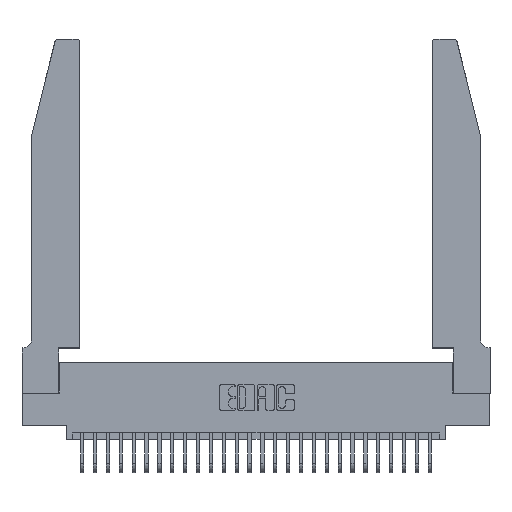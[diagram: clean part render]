
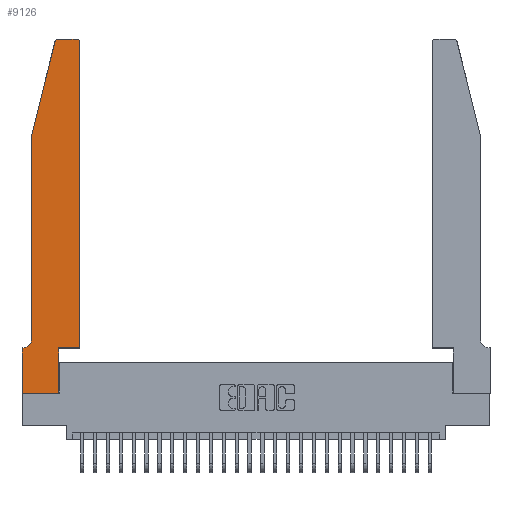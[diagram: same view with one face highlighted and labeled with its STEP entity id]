
A CAD part, top view. The second image highlights one B-rep face of the part: STEP entity #9126.
In plain terms, the highlighted planar face has unit normal (0, 0, 1).
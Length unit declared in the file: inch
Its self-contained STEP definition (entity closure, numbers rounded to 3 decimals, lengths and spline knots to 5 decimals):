
#20 = VECTOR ( 'NONE', #21429, 39.37008 ) ;
#166 = CARTESIAN_POINT ( 'NONE',  ( 0.284, 2.72, 0.37 ) ) ;
#540 = AXIS2_PLACEMENT_3D ( 'NONE', #166, #8974, #23031 ) ;
#569 = DIRECTION ( 'NONE',  ( -1., 0., 0. ) ) ;
#892 = LINE ( 'NONE', #29978, #26623 ) ;
#1623 = CIRCLE ( 'NONE', #21511, 0.03 ) ;
#2036 = CIRCLE ( 'NONE', #540, 0.03 ) ;
#2451 = DIRECTION ( 'NONE',  ( 0., 1., 0. ) ) ;
#2633 = EDGE_LOOP ( 'NONE', ( #7762, #2646, #11459, #7967, #24543, #28884, #22495, #23406, #10950, #25258, #8708, #3749 ) ) ;
#2646 = ORIENTED_EDGE ( 'NONE', *, *, #6330, .T. ) ;
#2944 = EDGE_CURVE ( 'NONE', #3368, #30185, #22848, .T. ) ;
#3368 = VERTEX_POINT ( 'NONE', #3520 ) ;
#3520 = CARTESIAN_POINT ( 'NONE',  ( 0.0755, 0.42, 0.37 ) ) ;
#3694 = LINE ( 'NONE', #16922, #20 ) ;
#3749 = ORIENTED_EDGE ( 'NONE', *, *, #21285, .T. ) ;
#3781 = CARTESIAN_POINT ( 'NONE',  ( 0.4505, 2.72, 0.37 ) ) ;
#3978 = VECTOR ( 'NONE', #569, 39.37008 ) ;
#5810 = EDGE_CURVE ( 'NONE', #25980, #11732, #6088, .T. ) ;
#6088 = LINE ( 'NONE', #26277, #10878 ) ;
#6330 = EDGE_CURVE ( 'NONE', #10317, #6847, #2036, .T. ) ;
#6740 = VECTOR ( 'NONE', #25103, 39.37008 ) ;
#6847 = VERTEX_POINT ( 'NONE', #18614 ) ;
#6936 = EDGE_CURVE ( 'NONE', #20469, #14770, #15983, .T. ) ;
#7747 = CARTESIAN_POINT ( 'NONE',  ( 0.2605, 2.75, 0.37 ) ) ;
#7762 = ORIENTED_EDGE ( 'NONE', *, *, #21442, .T. ) ;
#7824 = LINE ( 'NONE', #16456, #25850 ) ;
#7967 = ORIENTED_EDGE ( 'NONE', *, *, #21845, .T. ) ;
#8351 = VERTEX_POINT ( 'NONE', #26873 ) ;
#8708 = ORIENTED_EDGE ( 'NONE', *, *, #12063, .T. ) ;
#8974 = DIRECTION ( 'NONE',  ( 0., 0., 1. ) ) ;
#9126 = ADVANCED_FACE ( 'NONE', ( #10341 ), #14362, .T. ) ;
#9765 = CARTESIAN_POINT ( 'NONE',  ( 0.0055, 0.35, 0.37 ) ) ;
#10127 = EDGE_CURVE ( 'NONE', #14770, #8351, #7824, .T. ) ;
#10317 = VERTEX_POINT ( 'NONE', #12602 ) ;
#10341 = FACE_OUTER_BOUND ( 'NONE', #2633, .T. ) ;
#10596 = VERTEX_POINT ( 'NONE', #16826 ) ;
#10878 = VECTOR ( 'NONE', #23633, 39.37008 ) ;
#10950 = ORIENTED_EDGE ( 'NONE', *, *, #6936, .T. ) ;
#11459 = ORIENTED_EDGE ( 'NONE', *, *, #27651, .T. ) ;
#11683 = CARTESIAN_POINT ( 'NONE',  ( 0.4205, 2.72, 0.37 ) ) ;
#11732 = VERTEX_POINT ( 'NONE', #17463 ) ;
#12021 = CARTESIAN_POINT ( 'NONE',  ( 0.2865, 0.35, 0.37 ) ) ;
#12063 = EDGE_CURVE ( 'NONE', #8351, #26351, #3694, .T. ) ;
#12207 = CARTESIAN_POINT ( 'NONE',  ( 0.0755, 0.35, 0.37 ) ) ;
#12587 = DIRECTION ( 'NONE',  ( -1., 0., 0. ) ) ;
#12602 = CARTESIAN_POINT ( 'NONE',  ( 0.284, 2.75, 0.37 ) ) ;
#14362 = PLANE ( 'NONE',  #30348 ) ;
#14542 = VECTOR ( 'NONE', #28053, 39.37008 ) ;
#14770 = VERTEX_POINT ( 'NONE', #29901 ) ;
#15286 = EDGE_CURVE ( 'NONE', #11732, #20469, #18597, .T. ) ;
#15983 = LINE ( 'NONE', #12021, #19997 ) ;
#16456 = CARTESIAN_POINT ( 'NONE',  ( 0.4505, 0.35, 0.37 ) ) ;
#16826 = CARTESIAN_POINT ( 'NONE',  ( 0.0755, 2., 0.37 ) ) ;
#16922 = CARTESIAN_POINT ( 'NONE',  ( 0.4505, 0.35, 0.37 ) ) ;
#16949 = DIRECTION ( 'NONE',  ( 1., 0., 0. ) ) ;
#17057 = LINE ( 'NONE', #22947, #6740 ) ;
#17463 = CARTESIAN_POINT ( 'NONE',  ( 0., 0., 0.37 ) ) ;
#17955 = EDGE_CURVE ( 'NONE', #30185, #25980, #24205, .T. ) ;
#17999 = CARTESIAN_POINT ( 'NONE',  ( 0., 0.35, 0.37 ) ) ;
#18006 = CARTESIAN_POINT ( 'NONE',  ( 0.2865, 0., 0.37 ) ) ;
#18431 = CARTESIAN_POINT ( 'NONE',  ( 0.4205, 2.75, 0.37 ) ) ;
#18597 = LINE ( 'NONE', #21289, #14542 ) ;
#18614 = CARTESIAN_POINT ( 'NONE',  ( 0.25487, 2.72718, 0.37 ) ) ;
#18901 = LINE ( 'NONE', #7747, #19273 ) ;
#19273 = VECTOR ( 'NONE', #12587, 39.37008 ) ;
#19630 = VERTEX_POINT ( 'NONE', #18431 ) ;
#19997 = VECTOR ( 'NONE', #2451, 39.37008 ) ;
#20469 = VERTEX_POINT ( 'NONE', #18006 ) ;
#20734 = DIRECTION ( 'NONE',  ( 0., 0., 1. ) ) ;
#21285 = EDGE_CURVE ( 'NONE', #26351, #19630, #1623, .T. ) ;
#21289 = CARTESIAN_POINT ( 'NONE',  ( 0., 0., 0.37 ) ) ;
#21429 = DIRECTION ( 'NONE',  ( 0., 1., 0. ) ) ;
#21442 = EDGE_CURVE ( 'NONE', #19630, #10317, #18901, .T. ) ;
#21511 = AXIS2_PLACEMENT_3D ( 'NONE', #11683, #20734, #25461 ) ;
#21845 = EDGE_CURVE ( 'NONE', #10596, #3368, #17057, .T. ) ;
#22495 = ORIENTED_EDGE ( 'NONE', *, *, #5810, .T. ) ;
#22848 = CIRCLE ( 'NONE', #24316, 0.07 ) ;
#22947 = CARTESIAN_POINT ( 'NONE',  ( 0.0755, 2., 0.37 ) ) ;
#23031 = DIRECTION ( 'NONE',  ( 1., 0., 0. ) ) ;
#23226 = DIRECTION ( 'NONE',  ( -0.239, -0.971, 0. ) ) ;
#23406 = ORIENTED_EDGE ( 'NONE', *, *, #15286, .T. ) ;
#23613 = DIRECTION ( 'NONE',  ( 1., 0., 0. ) ) ;
#23633 = DIRECTION ( 'NONE',  ( 0., -1., 0. ) ) ;
#23917 = CARTESIAN_POINT ( 'NONE',  ( 0., 0.35, 0.37 ) ) ;
#24205 = LINE ( 'NONE', #12207, #3978 ) ;
#24316 = AXIS2_PLACEMENT_3D ( 'NONE', #29382, #27449, #27255 ) ;
#24543 = ORIENTED_EDGE ( 'NONE', *, *, #2944, .T. ) ;
#25103 = DIRECTION ( 'NONE',  ( 0., -1., 0. ) ) ;
#25258 = ORIENTED_EDGE ( 'NONE', *, *, #10127, .T. ) ;
#25461 = DIRECTION ( 'NONE',  ( 1., 0., 0. ) ) ;
#25850 = VECTOR ( 'NONE', #23613, 39.37008 ) ;
#25980 = VERTEX_POINT ( 'NONE', #17999 ) ;
#26263 = DIRECTION ( 'NONE',  ( 0., 0., 1. ) ) ;
#26277 = CARTESIAN_POINT ( 'NONE',  ( 0., 0., 0.37 ) ) ;
#26351 = VERTEX_POINT ( 'NONE', #3781 ) ;
#26623 = VECTOR ( 'NONE', #23226, 39.37008 ) ;
#26873 = CARTESIAN_POINT ( 'NONE',  ( 0.4505, 0.35, 0.37 ) ) ;
#27255 = DIRECTION ( 'NONE',  ( -1., 0., 0. ) ) ;
#27449 = DIRECTION ( 'NONE',  ( 0., 0., -1. ) ) ;
#27651 = EDGE_CURVE ( 'NONE', #6847, #10596, #892, .T. ) ;
#28053 = DIRECTION ( 'NONE',  ( 1., 0., 0. ) ) ;
#28884 = ORIENTED_EDGE ( 'NONE', *, *, #17955, .T. ) ;
#29382 = CARTESIAN_POINT ( 'NONE',  ( 0.0055, 0.42, 0.37 ) ) ;
#29901 = CARTESIAN_POINT ( 'NONE',  ( 0.2865, 0.35, 0.37 ) ) ;
#29978 = CARTESIAN_POINT ( 'NONE',  ( 0.0755, 2., 0.37 ) ) ;
#30185 = VERTEX_POINT ( 'NONE', #9765 ) ;
#30348 = AXIS2_PLACEMENT_3D ( 'NONE', #23917, #26263, #16949 ) ;
